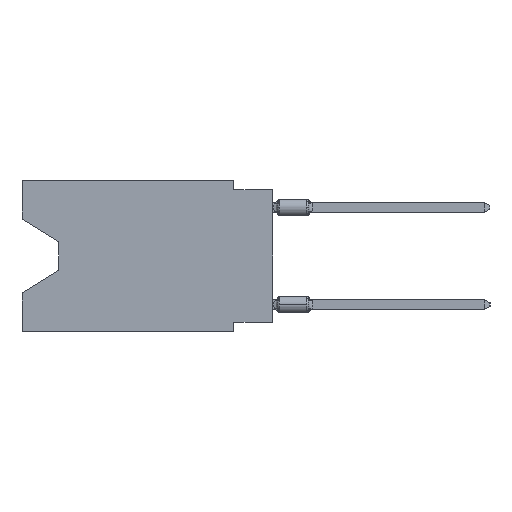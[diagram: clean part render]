
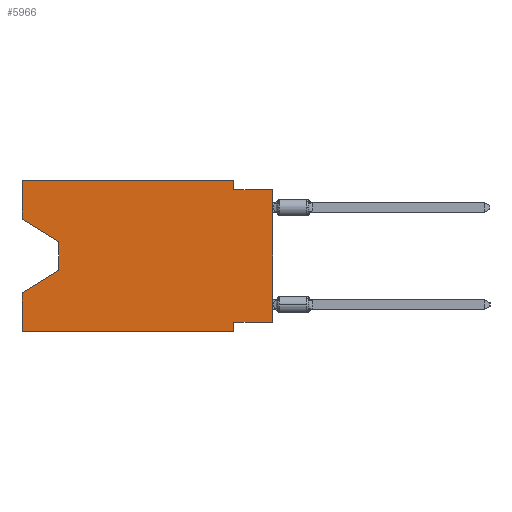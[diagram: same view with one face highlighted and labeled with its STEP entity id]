
A CAD part, left-side view. The second image highlights one B-rep face of the part: STEP entity #5966.
In plain terms, the highlighted planar face has unit normal (-1, 0, 0).
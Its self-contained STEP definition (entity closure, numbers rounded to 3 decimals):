
#1486 = DIRECTION ( 'NONE',  ( 0., 0., 1. ) ) ;
#1709 = LINE ( 'NONE', #6021, #60625 ) ;
#1968 = VERTEX_POINT ( 'NONE', #29727 ) ;
#2002 = DIRECTION ( 'NONE',  ( 0., -0.855, -0.519 ) ) ;
#2003 = CARTESIAN_POINT ( 'NONE',  ( 0., 16.383, 0. ) ) ;
#3118 = DIRECTION ( 'NONE',  ( 0., 1., 0. ) ) ;
#3418 = LINE ( 'NONE', #59541, #39637 ) ;
#3908 = ORIENTED_EDGE ( 'NONE', *, *, #27787, .F. ) ;
#5966 = ADVANCED_FACE ( 'NONE', ( #15520 ), #39439, .F. ) ;
#6021 = CARTESIAN_POINT ( 'NONE',  ( 0., 16.383, -2.546 ) ) ;
#7048 = VERTEX_POINT ( 'NONE', #46257 ) ;
#8038 = ORIENTED_EDGE ( 'NONE', *, *, #47019, .T. ) ;
#8625 = CARTESIAN_POINT ( 'NONE',  ( 0., 13.97, -4.013 ) ) ;
#8831 = ORIENTED_EDGE ( 'NONE', *, *, #49596, .T. ) ;
#10216 = VECTOR ( 'NONE', #17667, 1000. ) ;
#10999 = EDGE_CURVE ( 'NONE', #1968, #53004, #20955, .T. ) ;
#11631 = VERTEX_POINT ( 'NONE', #25356 ) ;
#11747 = DIRECTION ( 'NONE',  ( 0., 0., 1. ) ) ;
#12227 = DIRECTION ( 'NONE',  ( 0., 0.855, -0.519 ) ) ;
#12941 = EDGE_CURVE ( 'NONE', #24154, #39112, #3418, .T. ) ;
#13517 = DIRECTION ( 'NONE',  ( 0., 0., -1. ) ) ;
#14757 = EDGE_CURVE ( 'NONE', #29808, #11631, #38021, .T. ) ;
#15520 = FACE_OUTER_BOUND ( 'NONE', #16540, .T. ) ;
#16358 = CARTESIAN_POINT ( 'NONE',  ( 0., 16.383, 0. ) ) ;
#16540 = EDGE_LOOP ( 'NONE', ( #8831, #8038, #54978, #53587, #33452, #53291, #25587, #44714, #30483, #39127, #3908, #46928 ) ) ;
#17667 = DIRECTION ( 'NONE',  ( 0., -1., 0. ) ) ;
#18057 = AXIS2_PLACEMENT_3D ( 'NONE', #2003, #57231, #34835 ) ;
#19274 = VECTOR ( 'NONE', #13517, 1000. ) ;
#19604 = DIRECTION ( 'NONE',  ( 0., -1., 0. ) ) ;
#20955 = LINE ( 'NONE', #16358, #31494 ) ;
#22380 = CARTESIAN_POINT ( 'NONE',  ( 0., 13.97, -5.893 ) ) ;
#23375 = VECTOR ( 'NONE', #1486, 1000. ) ;
#24050 = DIRECTION ( 'NONE',  ( 0., -1., 0. ) ) ;
#24154 = VERTEX_POINT ( 'NONE', #27735 ) ;
#24183 = CARTESIAN_POINT ( 'NONE',  ( 0., 16.383, 0. ) ) ;
#24454 = VERTEX_POINT ( 'NONE', #24183 ) ;
#24955 = CARTESIAN_POINT ( 'NONE',  ( 0., 2.54, -9.906 ) ) ;
#25256 = DIRECTION ( 'NONE',  ( 0., 0., -1. ) ) ;
#25356 = CARTESIAN_POINT ( 'NONE',  ( 0., 0., -0.635 ) ) ;
#25587 = ORIENTED_EDGE ( 'NONE', *, *, #12941, .F. ) ;
#25819 = CARTESIAN_POINT ( 'NONE',  ( 0., 16.383, -7.36 ) ) ;
#26025 = CARTESIAN_POINT ( 'NONE',  ( 0., 2.54, -9.271 ) ) ;
#27735 = CARTESIAN_POINT ( 'NONE',  ( 0., 0., -9.271 ) ) ;
#27787 = EDGE_CURVE ( 'NONE', #24454, #7048, #33559, .T. ) ;
#29270 = LINE ( 'NONE', #24955, #46097 ) ;
#29727 = CARTESIAN_POINT ( 'NONE',  ( 0., 16.383, -9.906 ) ) ;
#29808 = VERTEX_POINT ( 'NONE', #49799 ) ;
#30010 = LINE ( 'NONE', #53612, #23375 ) ;
#30483 = ORIENTED_EDGE ( 'NONE', *, *, #14757, .F. ) ;
#31256 = CARTESIAN_POINT ( 'NONE',  ( 0., 13.97, -5.893 ) ) ;
#31483 = CARTESIAN_POINT ( 'NONE',  ( 0., 16.383, -9.906 ) ) ;
#31494 = VECTOR ( 'NONE', #11747, 1000. ) ;
#32546 = LINE ( 'NONE', #8625, #19274 ) ;
#32695 = CARTESIAN_POINT ( 'NONE',  ( 0., 16.383, -2.546 ) ) ;
#33452 = ORIENTED_EDGE ( 'NONE', *, *, #57980, .T. ) ;
#33548 = VECTOR ( 'NONE', #24050, 1000. ) ;
#33559 = LINE ( 'NONE', #43065, #33548 ) ;
#34637 = VERTEX_POINT ( 'NONE', #51685 ) ;
#34835 = DIRECTION ( 'NONE',  ( 0., 0., -1. ) ) ;
#35600 = EDGE_CURVE ( 'NONE', #51931, #53004, #57962, .T. ) ;
#36844 = EDGE_CURVE ( 'NONE', #39112, #49408, #29270, .T. ) ;
#37150 = LINE ( 'NONE', #50323, #38561 ) ;
#38021 = LINE ( 'NONE', #56715, #59216 ) ;
#38561 = VECTOR ( 'NONE', #56145, 1000. ) ;
#39112 = VERTEX_POINT ( 'NONE', #26025 ) ;
#39127 = ORIENTED_EDGE ( 'NONE', *, *, #55530, .F. ) ;
#39439 = PLANE ( 'NONE',  #18057 ) ;
#39637 = VECTOR ( 'NONE', #3118, 1000. ) ;
#43065 = CARTESIAN_POINT ( 'NONE',  ( 0., 16.383, 0. ) ) ;
#44478 = VECTOR ( 'NONE', #55383, 1000. ) ;
#44714 = ORIENTED_EDGE ( 'NONE', *, *, #49212, .T. ) ;
#45573 = LINE ( 'NONE', #31483, #10216 ) ;
#46097 = VECTOR ( 'NONE', #25256, 1000. ) ;
#46162 = CARTESIAN_POINT ( 'NONE',  ( 0., 16.383, 0. ) ) ;
#46257 = CARTESIAN_POINT ( 'NONE',  ( 0., 2.54, 0. ) ) ;
#46928 = ORIENTED_EDGE ( 'NONE', *, *, #58100, .F. ) ;
#47019 = EDGE_CURVE ( 'NONE', #34637, #51931, #32546, .T. ) ;
#49212 = EDGE_CURVE ( 'NONE', #24154, #11631, #30010, .T. ) ;
#49408 = VERTEX_POINT ( 'NONE', #53905 ) ;
#49463 = VERTEX_POINT ( 'NONE', #32695 ) ;
#49596 = EDGE_CURVE ( 'NONE', #49463, #34637, #1709, .T. ) ;
#49799 = CARTESIAN_POINT ( 'NONE',  ( 0., 2.54, -0.635 ) ) ;
#50323 = CARTESIAN_POINT ( 'NONE',  ( 0., 2.54, 0. ) ) ;
#50776 = LINE ( 'NONE', #46162, #44478 ) ;
#51685 = CARTESIAN_POINT ( 'NONE',  ( 0., 13.97, -4.013 ) ) ;
#51931 = VERTEX_POINT ( 'NONE', #22380 ) ;
#53004 = VERTEX_POINT ( 'NONE', #25819 ) ;
#53291 = ORIENTED_EDGE ( 'NONE', *, *, #36844, .F. ) ;
#53587 = ORIENTED_EDGE ( 'NONE', *, *, #10999, .F. ) ;
#53612 = CARTESIAN_POINT ( 'NONE',  ( 0., 0., 0. ) ) ;
#53626 = VECTOR ( 'NONE', #12227, 1000. ) ;
#53905 = CARTESIAN_POINT ( 'NONE',  ( 0., 2.54, -9.906 ) ) ;
#54978 = ORIENTED_EDGE ( 'NONE', *, *, #35600, .T. ) ;
#55383 = DIRECTION ( 'NONE',  ( 0., 0., 1. ) ) ;
#55530 = EDGE_CURVE ( 'NONE', #7048, #29808, #37150, .T. ) ;
#56145 = DIRECTION ( 'NONE',  ( 0., 0., -1. ) ) ;
#56715 = CARTESIAN_POINT ( 'NONE',  ( 0., 0., -0.635 ) ) ;
#57231 = DIRECTION ( 'NONE',  ( 1., 0., 0. ) ) ;
#57962 = LINE ( 'NONE', #31256, #53626 ) ;
#57980 = EDGE_CURVE ( 'NONE', #1968, #49408, #45573, .T. ) ;
#58100 = EDGE_CURVE ( 'NONE', #49463, #24454, #50776, .T. ) ;
#59216 = VECTOR ( 'NONE', #19604, 1000. ) ;
#59541 = CARTESIAN_POINT ( 'NONE',  ( 0., 0., -9.271 ) ) ;
#60625 = VECTOR ( 'NONE', #2002, 1000. ) ;
